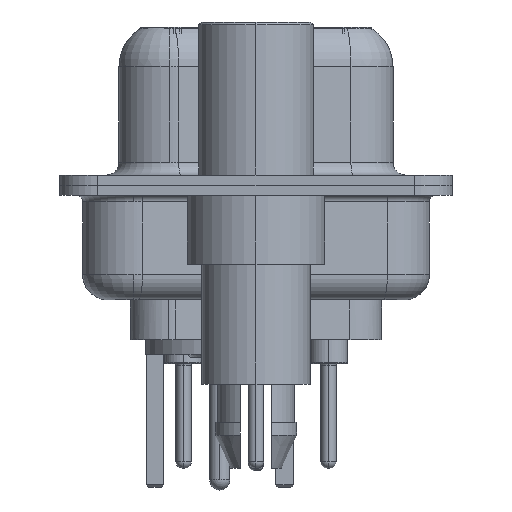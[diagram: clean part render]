
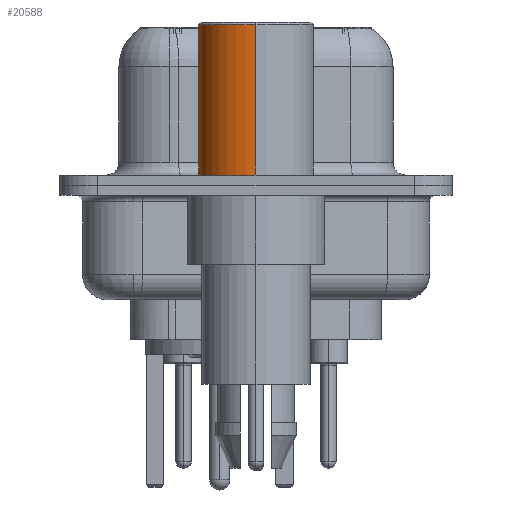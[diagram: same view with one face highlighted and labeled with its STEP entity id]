
A CAD part, left-side view. The second image highlights one B-rep face of the part: STEP entity #20588.
In plain terms, the highlighted cylindrical face has radius 2.25 mm (diameter 4.5 mm), a partial arc.
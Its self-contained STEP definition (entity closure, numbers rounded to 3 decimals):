
#1180 = DIRECTION ( 'NONE',  ( 0., 0., 1. ) ) ;
#2555 = CARTESIAN_POINT ( 'NONE',  ( 0., 0., 6.3 ) ) ;
#2682 = DIRECTION ( 'NONE',  ( 0., 0., 1. ) ) ;
#2777 = EDGE_CURVE ( 'NONE', #3570, #30261, #5844, .T. ) ;
#3570 = VERTEX_POINT ( 'NONE', #9574 ) ;
#4499 = AXIS2_PLACEMENT_3D ( 'NONE', #13255, #22021, #33154 ) ;
#4686 = ORIENTED_EDGE ( 'NONE', *, *, #10006, .F. ) ;
#5095 = DIRECTION ( 'NONE',  ( 1., 0., 0. ) ) ;
#5844 = CIRCLE ( 'NONE', #23907, 2.25 ) ;
#9574 = CARTESIAN_POINT ( 'NONE',  ( 2.25, 0., 0.4 ) ) ;
#9902 = VERTEX_POINT ( 'NONE', #16040 ) ;
#10006 = EDGE_CURVE ( 'NONE', #33287, #9902, #15979, .T. ) ;
#11609 = EDGE_CURVE ( 'NONE', #3570, #33287, #16463, .T. ) ;
#12673 = ORIENTED_EDGE ( 'NONE', *, *, #11609, .F. ) ;
#13255 = CARTESIAN_POINT ( 'NONE',  ( 0., 0., 0.581 ) ) ;
#15979 = CIRCLE ( 'NONE', #31724, 2.25 ) ;
#16007 = ORIENTED_EDGE ( 'NONE', *, *, #17533, .T. ) ;
#16040 = CARTESIAN_POINT ( 'NONE',  ( -2.25, 0., 6.3 ) ) ;
#16463 = LINE ( 'NONE', #17985, #35179 ) ;
#17261 = CYLINDRICAL_SURFACE ( 'NONE', #4499, 2.25 ) ;
#17533 = EDGE_CURVE ( 'NONE', #30261, #9902, #33272, .T. ) ;
#17985 = CARTESIAN_POINT ( 'NONE',  ( 2.25, 0., 0.581 ) ) ;
#19096 = DIRECTION ( 'NONE',  ( 1., 0., 0. ) ) ;
#19832 = DIRECTION ( 'NONE',  ( 0., 0., 1. ) ) ;
#20588 = ADVANCED_FACE ( 'NONE', ( #24671 ), #17261, .T. ) ;
#22021 = DIRECTION ( 'NONE',  ( 0., 0., 1. ) ) ;
#23907 = AXIS2_PLACEMENT_3D ( 'NONE', #33146, #27283, #19096 ) ;
#24671 = FACE_OUTER_BOUND ( 'NONE', #31873, .T. ) ;
#27283 = DIRECTION ( 'NONE',  ( 0., 0., 1. ) ) ;
#27470 = ORIENTED_EDGE ( 'NONE', *, *, #2777, .T. ) ;
#28150 = CARTESIAN_POINT ( 'NONE',  ( -2.25, 0., 0.581 ) ) ;
#28540 = CARTESIAN_POINT ( 'NONE',  ( -2.25, 0., 0.4 ) ) ;
#30261 = VERTEX_POINT ( 'NONE', #28540 ) ;
#31529 = VECTOR ( 'NONE', #19832, 1000. ) ;
#31699 = CARTESIAN_POINT ( 'NONE',  ( 2.25, 0., 6.3 ) ) ;
#31724 = AXIS2_PLACEMENT_3D ( 'NONE', #2555, #2682, #5095 ) ;
#31873 = EDGE_LOOP ( 'NONE', ( #27470, #16007, #4686, #12673 ) ) ;
#33146 = CARTESIAN_POINT ( 'NONE',  ( 0., 0., 0.4 ) ) ;
#33154 = DIRECTION ( 'NONE',  ( 1., 0., 0. ) ) ;
#33272 = LINE ( 'NONE', #28150, #31529 ) ;
#33287 = VERTEX_POINT ( 'NONE', #31699 ) ;
#35179 = VECTOR ( 'NONE', #1180, 1000. ) ;
